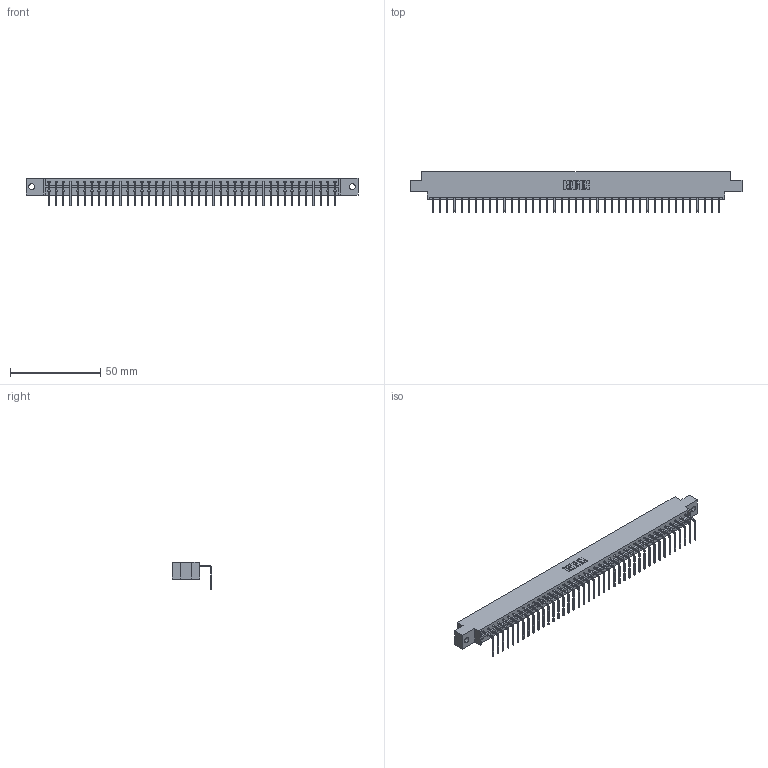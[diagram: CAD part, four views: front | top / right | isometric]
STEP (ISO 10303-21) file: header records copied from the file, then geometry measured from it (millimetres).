
FILE_DESCRIPTION (( 'STEP AP203' ), '1' );
FILE_NAME ('333-041-558-602.STEP', '2018-08-03T15:46:29', ( '' ), ( '' ), 'SwSTEP 2.0', 'SolidWorks 2016', '' );
FILE_SCHEMA (( 'CONFIG_CONTROL_DESIGN' ));
Length unit declared in the file: inch
Products named in the file (3): 333 Part_Offset - .128 Dia; 345-292-001_558 Tail - 2; 333-041-558-602
Assembly tree (42 placements, depth 2):
  333-041-558-602
    333 Part_Offset - .128 Dia
    345-292-001_558 Tail - 2  x41
Bounding box: 184 x 22.17 x 15.37 mm (x, y, z)
Volume: 18378.9 mm3; surface area: 20642.5 mm2
Topology: 42 solids, 42 shells, 2578 faces, 7785 edges, 5134 vertices
Faces by surface type: plane 1878, cylinder 700
Entity records: 25413 total; most frequent: CARTESIAN_POINT 4393, ORIENTED_EDGE 4370, DIRECTION 3707, EDGE_CURVE 2185, LINE 2057, VECTOR 2057, VERTEX_POINT 1454, AXIS2_PLACEMENT_3D 825
